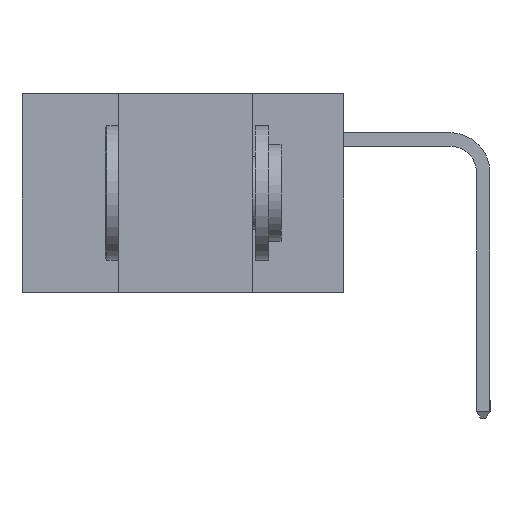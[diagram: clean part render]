
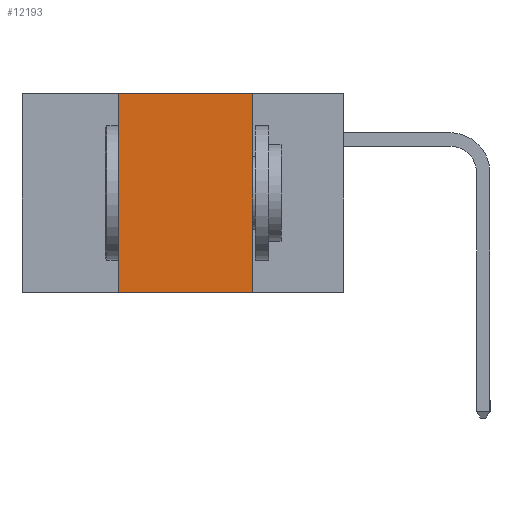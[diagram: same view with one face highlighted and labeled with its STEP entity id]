
A CAD part, left-side view. The second image highlights one B-rep face of the part: STEP entity #12193.
In plain terms, the highlighted planar face has unit normal (-1, 0, 0).
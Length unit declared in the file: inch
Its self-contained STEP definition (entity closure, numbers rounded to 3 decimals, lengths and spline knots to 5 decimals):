
#1252 = CARTESIAN_POINT ( 'NONE',  ( 0., 0.17, 0. ) ) ;
#2069 = PLANE ( 'NONE',  #12603 ) ;
#2132 = ORIENTED_EDGE ( 'NONE', *, *, #6909, .T. ) ;
#2589 = CARTESIAN_POINT ( 'NONE',  ( 0., 0.42, 0. ) ) ;
#4131 = EDGE_LOOP ( 'NONE', ( #13052, #9680, #9269, #2132 ) ) ;
#4212 = VECTOR ( 'NONE', #5552, 39.37008 ) ;
#4227 = EDGE_CURVE ( 'NONE', #9025, #7896, #14616, .T. ) ;
#4269 = DIRECTION ( 'NONE',  ( 0., 0., -1. ) ) ;
#4754 = DIRECTION ( 'NONE',  ( 1., 0., 0. ) ) ;
#4951 = LINE ( 'NONE', #9035, #14183 ) ;
#5024 = VECTOR ( 'NONE', #4269, 39.37008 ) ;
#5102 = EDGE_CURVE ( 'NONE', #6243, #9025, #4951, .T. ) ;
#5552 = DIRECTION ( 'NONE',  ( 0., -1., 0. ) ) ;
#6243 = VERTEX_POINT ( 'NONE', #13478 ) ;
#6909 = EDGE_CURVE ( 'NONE', #6243, #14843, #7779, .T. ) ;
#7386 = CARTESIAN_POINT ( 'NONE',  ( 0., 0.17, -0.37 ) ) ;
#7779 = LINE ( 'NONE', #12121, #4212 ) ;
#7896 = VERTEX_POINT ( 'NONE', #1252 ) ;
#8228 = FACE_OUTER_BOUND ( 'NONE', #4131, .T. ) ;
#8759 = CARTESIAN_POINT ( 'NONE',  ( 0., 0.6, 0. ) ) ;
#9025 = VERTEX_POINT ( 'NONE', #2589 ) ;
#9035 = CARTESIAN_POINT ( 'NONE',  ( 0., 0.42, -0.37 ) ) ;
#9236 = DIRECTION ( 'NONE',  ( 0., 0., 1. ) ) ;
#9269 = ORIENTED_EDGE ( 'NONE', *, *, #5102, .F. ) ;
#9680 = ORIENTED_EDGE ( 'NONE', *, *, #4227, .F. ) ;
#10906 = CARTESIAN_POINT ( 'NONE',  ( 0., 0.17, -0.37 ) ) ;
#11522 = DIRECTION ( 'NONE',  ( 0., -1., 0. ) ) ;
#11857 = CARTESIAN_POINT ( 'NONE',  ( 0., 0.6, 0. ) ) ;
#12121 = CARTESIAN_POINT ( 'NONE',  ( 0., 0.6, -0.37 ) ) ;
#12193 = ADVANCED_FACE ( 'NONE', ( #8228 ), #2069, .F. ) ;
#12603 = AXIS2_PLACEMENT_3D ( 'NONE', #8759, #4754, #13932 ) ;
#13052 = ORIENTED_EDGE ( 'NONE', *, *, #16718, .F. ) ;
#13478 = CARTESIAN_POINT ( 'NONE',  ( 0., 0.42, -0.37 ) ) ;
#13805 = VECTOR ( 'NONE', #11522, 39.37008 ) ;
#13932 = DIRECTION ( 'NONE',  ( 0., 0., -1. ) ) ;
#14183 = VECTOR ( 'NONE', #9236, 39.37008 ) ;
#14616 = LINE ( 'NONE', #11857, #13805 ) ;
#14843 = VERTEX_POINT ( 'NONE', #7386 ) ;
#15433 = LINE ( 'NONE', #10906, #5024 ) ;
#16718 = EDGE_CURVE ( 'NONE', #7896, #14843, #15433, .T. ) ;
